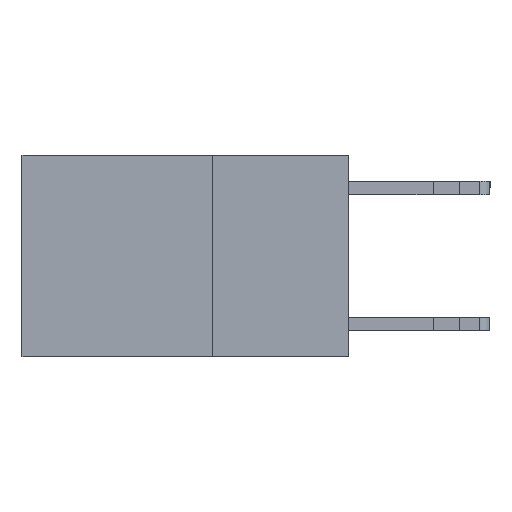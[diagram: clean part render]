
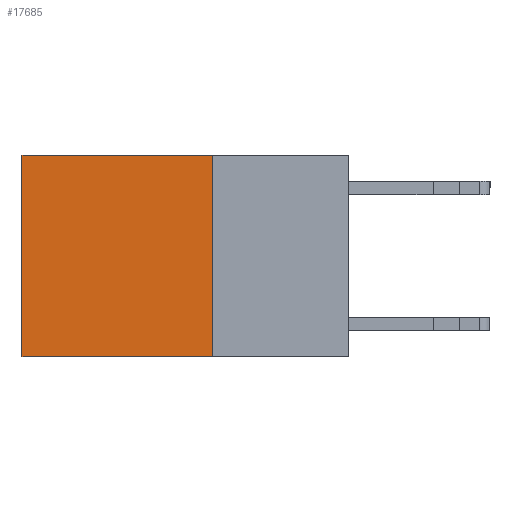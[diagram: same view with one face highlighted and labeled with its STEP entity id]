
A CAD part, left-side view. The second image highlights one B-rep face of the part: STEP entity #17685.
In plain terms, the highlighted planar face has unit normal (-1, 0, 0).
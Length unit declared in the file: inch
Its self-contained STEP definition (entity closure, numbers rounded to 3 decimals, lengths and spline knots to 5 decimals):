
#122 = CARTESIAN_POINT ( 'NONE',  ( 0.2625, 0.25, 0. ) ) ;
#557 = CARTESIAN_POINT ( 'NONE',  ( 0.2625, 0.6, -0.37 ) ) ;
#830 = LINE ( 'NONE', #4998, #9543 ) ;
#1413 = CARTESIAN_POINT ( 'NONE',  ( 0.2625, 0.6, 0. ) ) ;
#1596 = LINE ( 'NONE', #2791, #13197 ) ;
#1854 = ORIENTED_EDGE ( 'NONE', *, *, #10957, .F. ) ;
#2791 = CARTESIAN_POINT ( 'NONE',  ( 0.2625, 0.25, -0.37 ) ) ;
#3162 = VERTEX_POINT ( 'NONE', #557 ) ;
#4073 = VERTEX_POINT ( 'NONE', #8198 ) ;
#4304 = EDGE_LOOP ( 'NONE', ( #18772, #1854, #7410, #16038 ) ) ;
#4936 = LINE ( 'NONE', #18616, #8614 ) ;
#4998 = CARTESIAN_POINT ( 'NONE',  ( 0.2625, 0.25, 0. ) ) ;
#5446 = CARTESIAN_POINT ( 'NONE',  ( 0.2625, 0.25, 0. ) ) ;
#6420 = DIRECTION ( 'NONE',  ( 0., 0., -1. ) ) ;
#7410 = ORIENTED_EDGE ( 'NONE', *, *, #18630, .F. ) ;
#7927 = AXIS2_PLACEMENT_3D ( 'NONE', #19320, #14956, #16621 ) ;
#7956 = LINE ( 'NONE', #122, #10428 ) ;
#8198 = CARTESIAN_POINT ( 'NONE',  ( 0.2625, 0.25, -0.37 ) ) ;
#8614 = VECTOR ( 'NONE', #6420, 39.37008 ) ;
#9543 = VECTOR ( 'NONE', #15702, 39.37008 ) ;
#10428 = VECTOR ( 'NONE', #12108, 39.37008 ) ;
#10957 = EDGE_CURVE ( 'NONE', #4073, #3162, #1596, .T. ) ;
#11570 = FACE_OUTER_BOUND ( 'NONE', #4304, .T. ) ;
#12108 = DIRECTION ( 'NONE',  ( 0., 1., 0. ) ) ;
#13197 = VECTOR ( 'NONE', #16669, 39.37008 ) ;
#14956 = DIRECTION ( 'NONE',  ( 1., 0., 0. ) ) ;
#15702 = DIRECTION ( 'NONE',  ( 0., 0., -1. ) ) ;
#15940 = PLANE ( 'NONE',  #7927 ) ;
#16038 = ORIENTED_EDGE ( 'NONE', *, *, #16346, .T. ) ;
#16346 = EDGE_CURVE ( 'NONE', #18952, #16919, #7956, .T. ) ;
#16621 = DIRECTION ( 'NONE',  ( 0., 0., -1. ) ) ;
#16669 = DIRECTION ( 'NONE',  ( 0., 1., 0. ) ) ;
#16717 = EDGE_CURVE ( 'NONE', #16919, #3162, #4936, .T. ) ;
#16919 = VERTEX_POINT ( 'NONE', #1413 ) ;
#17685 = ADVANCED_FACE ( 'NONE', ( #11570 ), #15940, .F. ) ;
#18616 = CARTESIAN_POINT ( 'NONE',  ( 0.2625, 0.6, 0. ) ) ;
#18630 = EDGE_CURVE ( 'NONE', #18952, #4073, #830, .T. ) ;
#18772 = ORIENTED_EDGE ( 'NONE', *, *, #16717, .T. ) ;
#18952 = VERTEX_POINT ( 'NONE', #5446 ) ;
#19320 = CARTESIAN_POINT ( 'NONE',  ( 0.2625, 0.25, 0. ) ) ;
